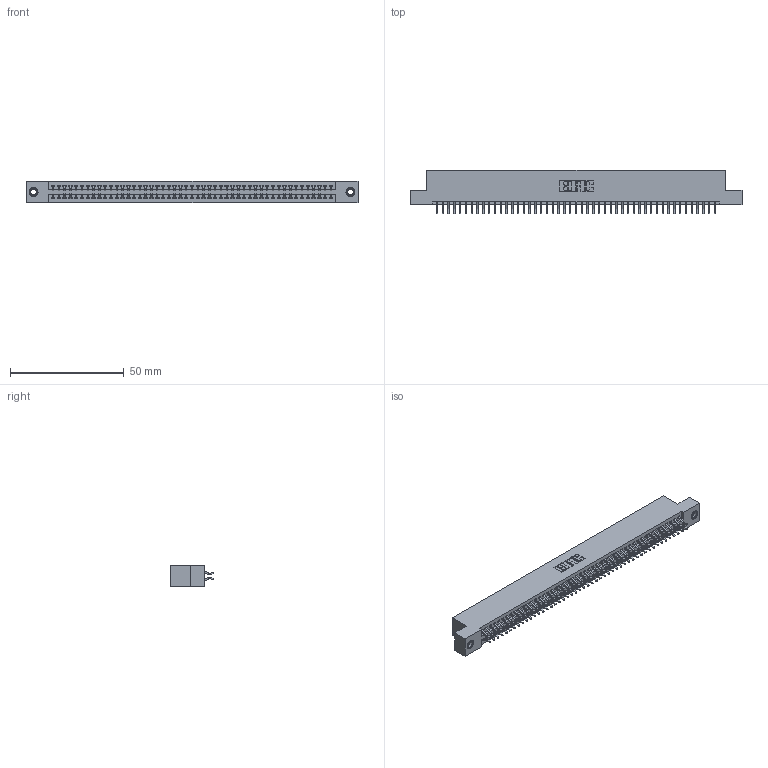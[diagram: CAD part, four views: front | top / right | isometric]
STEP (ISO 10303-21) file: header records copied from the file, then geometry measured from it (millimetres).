
FILE_DESCRIPTION (( 'STEP AP203' ), '1' );
FILE_NAME ('345-098-556-207.STEP', '2019-11-02T12:39:05', ( '' ), ( '' ), 'SwSTEP 2.0', 'SolidWorks 2016', '' );
FILE_SCHEMA (( 'CONFIG_CONTROL_DESIGN' ));
Length unit declared in the file: inch
Products named in the file (4): 345 Part_Flush Mounting Lugs - 0.156 Dia-TI; 345-250-001_345-250-005-103; 345-098-556-207; 345-292-001_556 Tail
Assembly tree (101 placements, depth 2):
  345-098-556-207
    345 Part_Flush Mounting Lugs - 0.156 Dia-TI
    345-292-001_556 Tail  x98
    345-250-001_345-250-005-103  x2
Bounding box: 145.67 x 19.24 x 9.4 mm (x, y, z)
Volume: 14198 mm3; surface area: 21064.7 mm2
Topology: 101 solids, 101 shells, 5674 faces, 16843 edges, 11090 vertices
Faces by surface type: plane 3738, cylinder 1920, cone 12, torus 4
Entity records: 38910 total; most frequent: CARTESIAN_POINT 6511, ORIENTED_EDGE 6426, DIRECTION 5747, EDGE_CURVE 3213, VECTOR 2857, LINE 2857, VERTEX_POINT 2136, AXIS2_PLACEMENT_3D 1445
